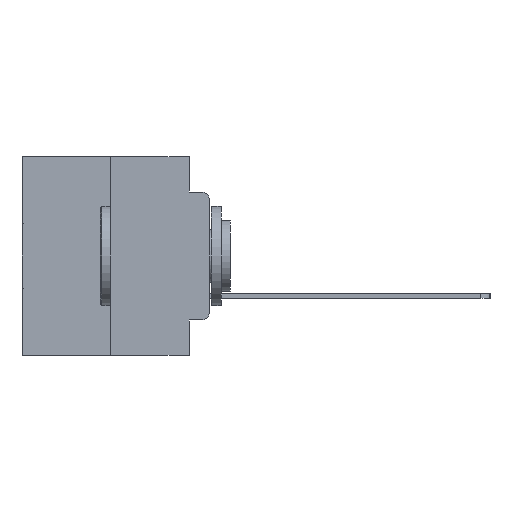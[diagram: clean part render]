
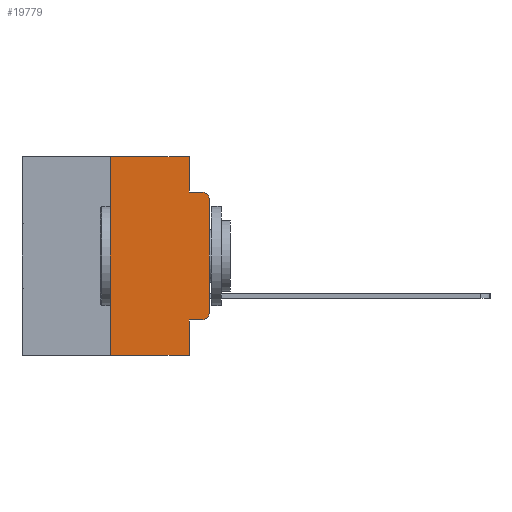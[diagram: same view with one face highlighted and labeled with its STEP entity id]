
A CAD part, left-side view. The second image highlights one B-rep face of the part: STEP entity #19779.
In plain terms, the highlighted planar face has unit normal (-1, 0, 0).
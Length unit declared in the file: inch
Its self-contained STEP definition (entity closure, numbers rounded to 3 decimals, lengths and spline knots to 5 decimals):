
#491 = ORIENTED_EDGE ( 'NONE', *, *, #22888, .F. ) ;
#608 = DIRECTION ( 'NONE',  ( 0., 0., -1. ) ) ;
#982 = DIRECTION ( 'NONE',  ( 0., 0., 1. ) ) ;
#1045 = EDGE_CURVE ( 'NONE', #19679, #27141, #23484, .T. ) ;
#1428 = FACE_OUTER_BOUND ( 'NONE', #7827, .T. ) ;
#1568 = LINE ( 'NONE', #22757, #6616 ) ;
#1681 = EDGE_CURVE ( 'NONE', #10970, #5391, #3905, .T. ) ;
#1816 = VECTOR ( 'NONE', #13204, 39.37008 ) ;
#2251 = CARTESIAN_POINT ( 'NONE',  ( 0., 0.25, 0. ) ) ;
#2609 = DIRECTION ( 'NONE',  ( 0., 0., -1. ) ) ;
#3140 = VECTOR ( 'NONE', #9114, 39.37008 ) ;
#3368 = EDGE_CURVE ( 'NONE', #10970, #21034, #20448, .T. ) ;
#3905 = LINE ( 'NONE', #25654, #3140 ) ;
#4072 = ORIENTED_EDGE ( 'NONE', *, *, #18623, .T. ) ;
#4333 = VERTEX_POINT ( 'NONE', #2251 ) ;
#5097 = DIRECTION ( 'NONE',  ( -1., 0., 0. ) ) ;
#5391 = VERTEX_POINT ( 'NONE', #29276 ) ;
#5552 = DIRECTION ( 'NONE',  ( 0., -1., 0. ) ) ;
#6039 = CARTESIAN_POINT ( 'NONE',  ( 0., 0.051, -0.0885 ) ) ;
#6197 = CARTESIAN_POINT ( 'NONE',  ( 0., 0.051, -0.4115 ) ) ;
#6616 = VECTOR ( 'NONE', #982, 39.37008 ) ;
#6711 = DIRECTION ( 'NONE',  ( 0., -1., 0. ) ) ;
#7374 = AXIS2_PLACEMENT_3D ( 'NONE', #28457, #21706, #7381 ) ;
#7381 = DIRECTION ( 'NONE',  ( 0., 0., -1. ) ) ;
#7827 = EDGE_LOOP ( 'NONE', ( #21770, #17737, #30029, #24684, #491, #9495, #28989, #24331, #22506, #4072 ) ) ;
#8067 = VECTOR ( 'NONE', #25758, 39.37008 ) ;
#8371 = EDGE_CURVE ( 'NONE', #9566, #4333, #1568, .T. ) ;
#8608 = CARTESIAN_POINT ( 'NONE',  ( 0., 0.25, -0.5 ) ) ;
#8660 = CARTESIAN_POINT ( 'NONE',  ( 0., 0., 0. ) ) ;
#8835 = EDGE_CURVE ( 'NONE', #9566, #21034, #17945, .T. ) ;
#9035 = CIRCLE ( 'NONE', #21553, 0.02 ) ;
#9108 = DIRECTION ( 'NONE',  ( 0., 0., 1. ) ) ;
#9114 = DIRECTION ( 'NONE',  ( 0., -1., 0. ) ) ;
#9495 = ORIENTED_EDGE ( 'NONE', *, *, #8371, .F. ) ;
#9566 = VERTEX_POINT ( 'NONE', #8608 ) ;
#10171 = VERTEX_POINT ( 'NONE', #29634 ) ;
#10479 = CARTESIAN_POINT ( 'NONE',  ( 0., 0.473, -0.5 ) ) ;
#10753 = LINE ( 'NONE', #19575, #28699 ) ;
#10970 = VERTEX_POINT ( 'NONE', #6197 ) ;
#11457 = AXIS2_PLACEMENT_3D ( 'NONE', #19624, #5097, #21966 ) ;
#12098 = CARTESIAN_POINT ( 'NONE',  ( 0., 0., -0.1085 ) ) ;
#13190 = EDGE_CURVE ( 'NONE', #10171, #25360, #10753, .T. ) ;
#13204 = DIRECTION ( 'NONE',  ( 0., 0., -1. ) ) ;
#14463 = LINE ( 'NONE', #25663, #8067 ) ;
#14877 = CARTESIAN_POINT ( 'NONE',  ( 0., 0.051, -0.5 ) ) ;
#15314 = DIRECTION ( 'NONE',  ( -1., 0., 0. ) ) ;
#16301 = CARTESIAN_POINT ( 'NONE',  ( 0., 0.473, 0. ) ) ;
#17180 = VECTOR ( 'NONE', #5552, 39.37008 ) ;
#17737 = ORIENTED_EDGE ( 'NONE', *, *, #27369, .T. ) ;
#17945 = LINE ( 'NONE', #10479, #17180 ) ;
#18320 = CARTESIAN_POINT ( 'NONE',  ( 0., 0.02, -0.0885 ) ) ;
#18623 = EDGE_CURVE ( 'NONE', #5391, #19679, #28427, .T. ) ;
#19371 = PLANE ( 'NONE',  #7374 ) ;
#19575 = CARTESIAN_POINT ( 'NONE',  ( 0., 0.051, 0. ) ) ;
#19613 = EDGE_CURVE ( 'NONE', #25360, #30816, #14463, .T. ) ;
#19624 = CARTESIAN_POINT ( 'NONE',  ( 0., 0.02, -0.3915 ) ) ;
#19679 = VERTEX_POINT ( 'NONE', #28246 ) ;
#19779 = ADVANCED_FACE ( 'NONE', ( #1428 ), #19371, .F. ) ;
#20448 = LINE ( 'NONE', #29557, #1816 ) ;
#21034 = VERTEX_POINT ( 'NONE', #14877 ) ;
#21553 = AXIS2_PLACEMENT_3D ( 'NONE', #29289, #15314, #608 ) ;
#21706 = DIRECTION ( 'NONE',  ( 1., 0., 0. ) ) ;
#21770 = ORIENTED_EDGE ( 'NONE', *, *, #1045, .T. ) ;
#21966 = DIRECTION ( 'NONE',  ( 0., 0., -1. ) ) ;
#22045 = VECTOR ( 'NONE', #9108, 39.37008 ) ;
#22506 = ORIENTED_EDGE ( 'NONE', *, *, #1681, .T. ) ;
#22757 = CARTESIAN_POINT ( 'NONE',  ( 0., 0.25, 0. ) ) ;
#22888 = EDGE_CURVE ( 'NONE', #4333, #10171, #30474, .T. ) ;
#23484 = LINE ( 'NONE', #8660, #22045 ) ;
#24331 = ORIENTED_EDGE ( 'NONE', *, *, #3368, .F. ) ;
#24405 = VECTOR ( 'NONE', #6711, 39.37008 ) ;
#24684 = ORIENTED_EDGE ( 'NONE', *, *, #13190, .F. ) ;
#25360 = VERTEX_POINT ( 'NONE', #6039 ) ;
#25654 = CARTESIAN_POINT ( 'NONE',  ( 0., 0.051, -0.4115 ) ) ;
#25663 = CARTESIAN_POINT ( 'NONE',  ( 0., 0.051, -0.0885 ) ) ;
#25758 = DIRECTION ( 'NONE',  ( 0., -1., 0. ) ) ;
#27141 = VERTEX_POINT ( 'NONE', #12098 ) ;
#27369 = EDGE_CURVE ( 'NONE', #27141, #30816, #9035, .T. ) ;
#28246 = CARTESIAN_POINT ( 'NONE',  ( 0., 0., -0.3915 ) ) ;
#28427 = CIRCLE ( 'NONE', #11457, 0.02 ) ;
#28457 = CARTESIAN_POINT ( 'NONE',  ( 0., 0.473, 0. ) ) ;
#28699 = VECTOR ( 'NONE', #2609, 39.37008 ) ;
#28989 = ORIENTED_EDGE ( 'NONE', *, *, #8835, .T. ) ;
#29276 = CARTESIAN_POINT ( 'NONE',  ( 0., 0.02, -0.4115 ) ) ;
#29289 = CARTESIAN_POINT ( 'NONE',  ( 0., 0.02, -0.1085 ) ) ;
#29557 = CARTESIAN_POINT ( 'NONE',  ( 0., 0.051, 0. ) ) ;
#29634 = CARTESIAN_POINT ( 'NONE',  ( 0., 0.051, 0. ) ) ;
#30029 = ORIENTED_EDGE ( 'NONE', *, *, #19613, .F. ) ;
#30474 = LINE ( 'NONE', #16301, #24405 ) ;
#30816 = VERTEX_POINT ( 'NONE', #18320 ) ;
